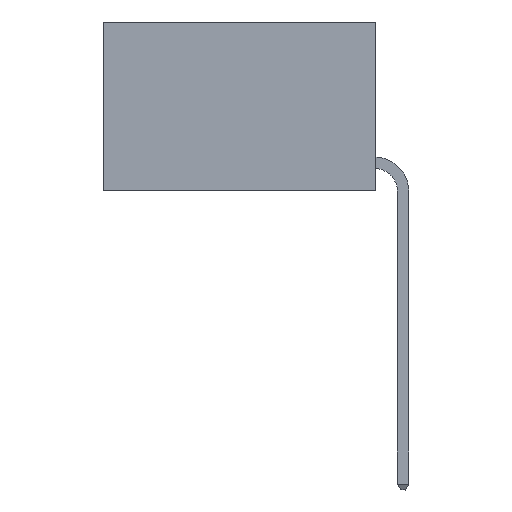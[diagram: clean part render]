
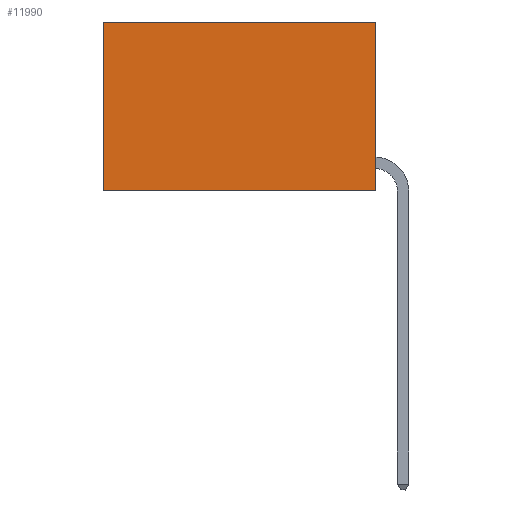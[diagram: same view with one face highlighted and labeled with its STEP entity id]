
A CAD part, left-side view. The second image highlights one B-rep face of the part: STEP entity #11990.
In plain terms, the highlighted planar face has unit normal (-1, 0, 0).
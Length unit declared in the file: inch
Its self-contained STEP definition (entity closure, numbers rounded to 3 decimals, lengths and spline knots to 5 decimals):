
#285 = EDGE_LOOP ( 'NONE', ( #12225, #3933, #3786, #24358 ) ) ;
#2944 = DIRECTION ( 'NONE',  ( 0., 0., -1. ) ) ;
#3726 = VECTOR ( 'NONE', #2944, 39.37008 ) ;
#3786 = ORIENTED_EDGE ( 'NONE', *, *, #5141, .F. ) ;
#3827 = CARTESIAN_POINT ( 'NONE',  ( 0.2625, 0.6, 0. ) ) ;
#3933 = ORIENTED_EDGE ( 'NONE', *, *, #5110, .F. ) ;
#5110 = EDGE_CURVE ( 'NONE', #9826, #26824, #24829, .T. ) ;
#5141 = EDGE_CURVE ( 'NONE', #16401, #9826, #13130, .T. ) ;
#5143 = CARTESIAN_POINT ( 'NONE',  ( 0.2625, 0.6, 0. ) ) ;
#6410 = PLANE ( 'NONE',  #20183 ) ;
#7077 = DIRECTION ( 'NONE',  ( 0., 1., 0. ) ) ;
#8086 = VECTOR ( 'NONE', #19770, 39.37008 ) ;
#9151 = FACE_OUTER_BOUND ( 'NONE', #285, .T. ) ;
#9186 = LINE ( 'NONE', #21916, #26477 ) ;
#9475 = LINE ( 'NONE', #5143, #3726 ) ;
#9826 = VERTEX_POINT ( 'NONE', #21667 ) ;
#10720 = DIRECTION ( 'NONE',  ( 1., 0., 0. ) ) ;
#11463 = DIRECTION ( 'NONE',  ( 0., 1., 0. ) ) ;
#11505 = CARTESIAN_POINT ( 'NONE',  ( 0.2625, 0., 0. ) ) ;
#11990 = ADVANCED_FACE ( 'NONE', ( #9151 ), #6410, .F. ) ;
#12225 = ORIENTED_EDGE ( 'NONE', *, *, #24179, .T. ) ;
#13130 = LINE ( 'NONE', #19860, #8086 ) ;
#13796 = VECTOR ( 'NONE', #7077, 39.37008 ) ;
#13898 = VERTEX_POINT ( 'NONE', #3827 ) ;
#16401 = VERTEX_POINT ( 'NONE', #11505 ) ;
#18975 = CARTESIAN_POINT ( 'NONE',  ( 0.2625, 0.6, -0.37 ) ) ;
#19770 = DIRECTION ( 'NONE',  ( 0., 0., -1. ) ) ;
#19860 = CARTESIAN_POINT ( 'NONE',  ( 0.2625, 0., 0. ) ) ;
#20183 = AXIS2_PLACEMENT_3D ( 'NONE', #21211, #10720, #25316 ) ;
#21211 = CARTESIAN_POINT ( 'NONE',  ( 0.2625, 0., 0. ) ) ;
#21667 = CARTESIAN_POINT ( 'NONE',  ( 0.2625, 0., -0.37 ) ) ;
#21844 = CARTESIAN_POINT ( 'NONE',  ( 0.2625, 0., -0.37 ) ) ;
#21916 = CARTESIAN_POINT ( 'NONE',  ( 0.2625, 0., 0. ) ) ;
#23571 = EDGE_CURVE ( 'NONE', #16401, #13898, #9186, .T. ) ;
#24179 = EDGE_CURVE ( 'NONE', #13898, #26824, #9475, .T. ) ;
#24358 = ORIENTED_EDGE ( 'NONE', *, *, #23571, .T. ) ;
#24829 = LINE ( 'NONE', #21844, #13796 ) ;
#25316 = DIRECTION ( 'NONE',  ( 0., 0., -1. ) ) ;
#26477 = VECTOR ( 'NONE', #11463, 39.37008 ) ;
#26824 = VERTEX_POINT ( 'NONE', #18975 ) ;
